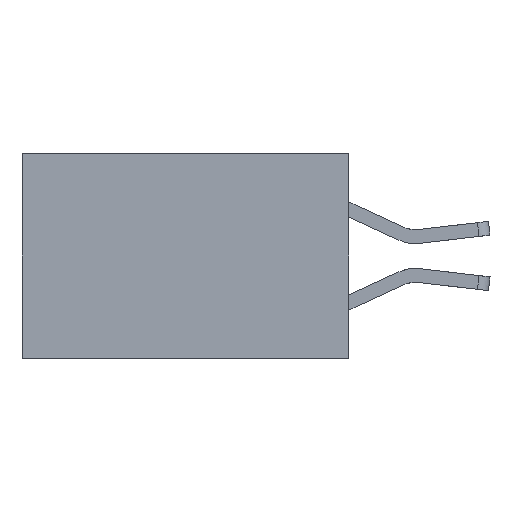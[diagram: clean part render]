
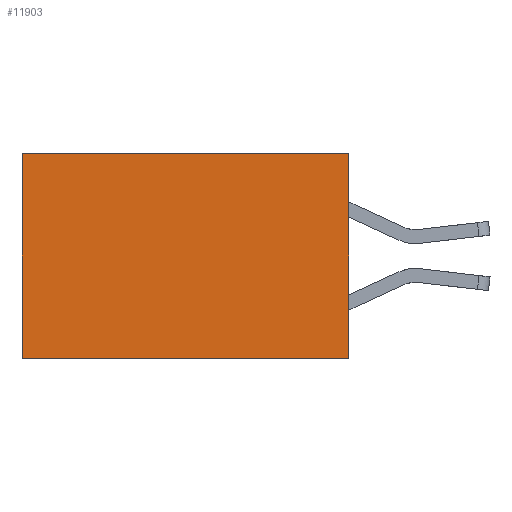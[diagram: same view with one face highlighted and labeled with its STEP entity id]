
A CAD part, left-side view. The second image highlights one B-rep face of the part: STEP entity #11903.
In plain terms, the highlighted planar face has unit normal (-1, 0, 0).
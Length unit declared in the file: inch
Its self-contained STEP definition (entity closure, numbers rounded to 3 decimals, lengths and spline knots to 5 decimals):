
#363 = DIRECTION ( 'NONE',  ( 0., 0., -1. ) ) ;
#551 = AXIS2_PLACEMENT_3D ( 'NONE', #14386, #7468, #363 ) ;
#641 = DIRECTION ( 'NONE',  ( 0., 1., 0. ) ) ;
#663 = CARTESIAN_POINT ( 'NONE',  ( 0.277, 0., -0.37 ) ) ;
#1252 = VERTEX_POINT ( 'NONE', #1781 ) ;
#1376 = CARTESIAN_POINT ( 'NONE',  ( 0.277, 0., 0. ) ) ;
#1653 = VERTEX_POINT ( 'NONE', #5879 ) ;
#1760 = LINE ( 'NONE', #663, #10181 ) ;
#1781 = CARTESIAN_POINT ( 'NONE',  ( 0.277, 0.59, 0. ) ) ;
#2293 = CARTESIAN_POINT ( 'NONE',  ( 0.277, 0., -0.37 ) ) ;
#2537 = FACE_OUTER_BOUND ( 'NONE', #2590, .T. ) ;
#2590 = EDGE_LOOP ( 'NONE', ( #12092, #9085, #3522, #6645 ) ) ;
#3522 = ORIENTED_EDGE ( 'NONE', *, *, #9859, .F. ) ;
#3695 = VECTOR ( 'NONE', #7026, 39.37008 ) ;
#3869 = EDGE_CURVE ( 'NONE', #8023, #1252, #4250, .T. ) ;
#4250 = LINE ( 'NONE', #1376, #10039 ) ;
#5634 = EDGE_CURVE ( 'NONE', #1653, #14213, #1760, .T. ) ;
#5879 = CARTESIAN_POINT ( 'NONE',  ( 0.277, 0., -0.37 ) ) ;
#6297 = PLANE ( 'NONE',  #551 ) ;
#6645 = ORIENTED_EDGE ( 'NONE', *, *, #3869, .T. ) ;
#6922 = CARTESIAN_POINT ( 'NONE',  ( 0.277, 0.59, -0.37 ) ) ;
#7026 = DIRECTION ( 'NONE',  ( 0., 0., -1. ) ) ;
#7468 = DIRECTION ( 'NONE',  ( 1., 0., 0. ) ) ;
#7554 = VECTOR ( 'NONE', #10453, 39.37008 ) ;
#8023 = VERTEX_POINT ( 'NONE', #13425 ) ;
#9085 = ORIENTED_EDGE ( 'NONE', *, *, #5634, .F. ) ;
#9859 = EDGE_CURVE ( 'NONE', #8023, #1653, #10630, .T. ) ;
#9883 = EDGE_CURVE ( 'NONE', #1252, #14213, #12993, .T. ) ;
#10039 = VECTOR ( 'NONE', #12491, 39.37008 ) ;
#10181 = VECTOR ( 'NONE', #641, 39.37008 ) ;
#10453 = DIRECTION ( 'NONE',  ( 0., 0., -1. ) ) ;
#10630 = LINE ( 'NONE', #2293, #7554 ) ;
#11224 = CARTESIAN_POINT ( 'NONE',  ( 0.277, 0.59, -0.37 ) ) ;
#11903 = ADVANCED_FACE ( 'NONE', ( #2537 ), #6297, .F. ) ;
#12092 = ORIENTED_EDGE ( 'NONE', *, *, #9883, .T. ) ;
#12491 = DIRECTION ( 'NONE',  ( 0., 1., 0. ) ) ;
#12993 = LINE ( 'NONE', #6922, #3695 ) ;
#13425 = CARTESIAN_POINT ( 'NONE',  ( 0.277, 0., 0. ) ) ;
#14213 = VERTEX_POINT ( 'NONE', #11224 ) ;
#14386 = CARTESIAN_POINT ( 'NONE',  ( 0.277, 0., -0.37 ) ) ;
